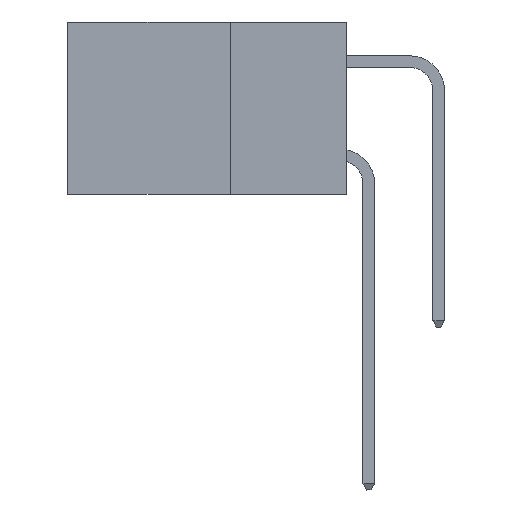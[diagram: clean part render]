
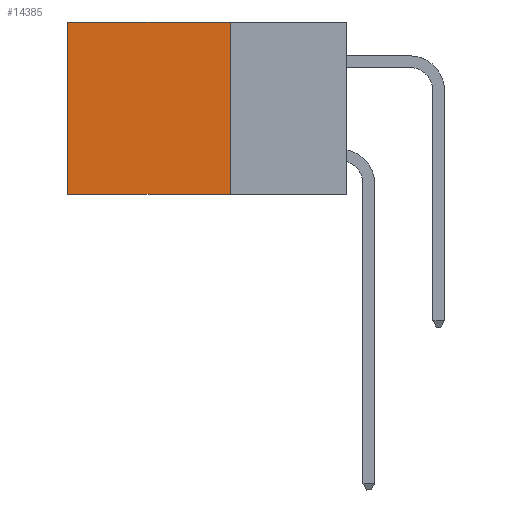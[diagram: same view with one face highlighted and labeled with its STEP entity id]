
A CAD part, left-side view. The second image highlights one B-rep face of the part: STEP entity #14385.
In plain terms, the highlighted planar face has unit normal (-1, 0, 0).
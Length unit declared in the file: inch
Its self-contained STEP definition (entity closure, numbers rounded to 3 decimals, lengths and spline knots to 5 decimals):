
#94 = CARTESIAN_POINT ( 'NONE',  ( 0.2875, 0.25, 0. ) ) ;
#2860 = DIRECTION ( 'NONE',  ( 0., 0., -1. ) ) ;
#2896 = ORIENTED_EDGE ( 'NONE', *, *, #21479, .T. ) ;
#3396 = EDGE_CURVE ( 'NONE', #15902, #11351, #21420, .T. ) ;
#3642 = DIRECTION ( 'NONE',  ( 0., 1., 0. ) ) ;
#4456 = CARTESIAN_POINT ( 'NONE',  ( 0.2875, 0.25, 0. ) ) ;
#4627 = CARTESIAN_POINT ( 'NONE',  ( 0.2875, 0.6, 0. ) ) ;
#4757 = VERTEX_POINT ( 'NONE', #4627 ) ;
#4791 = CARTESIAN_POINT ( 'NONE',  ( 0.2875, 0.25, -0.37 ) ) ;
#4839 = VERTEX_POINT ( 'NONE', #94 ) ;
#5002 = AXIS2_PLACEMENT_3D ( 'NONE', #4456, #22032, #11767 ) ;
#5581 = EDGE_LOOP ( 'NONE', ( #2896, #14275, #15285, #17978 ) ) ;
#5645 = LINE ( 'NONE', #17082, #9320 ) ;
#6939 = CARTESIAN_POINT ( 'NONE',  ( 0.2875, 0.25, 0. ) ) ;
#8459 = EDGE_CURVE ( 'NONE', #4839, #15902, #5645, .T. ) ;
#8718 = DIRECTION ( 'NONE',  ( 0., 1., 0. ) ) ;
#9116 = CARTESIAN_POINT ( 'NONE',  ( 0.2875, 0.25, -0.37 ) ) ;
#9320 = VECTOR ( 'NONE', #2860, 39.37008 ) ;
#9690 = CARTESIAN_POINT ( 'NONE',  ( 0.2875, 0.6, 0. ) ) ;
#9973 = PLANE ( 'NONE',  #5002 ) ;
#10730 = LINE ( 'NONE', #6939, #19358 ) ;
#11351 = VERTEX_POINT ( 'NONE', #12618 ) ;
#11506 = DIRECTION ( 'NONE',  ( 0., 0., -1. ) ) ;
#11767 = DIRECTION ( 'NONE',  ( 0., 0., -1. ) ) ;
#12109 = VECTOR ( 'NONE', #11506, 39.37008 ) ;
#12618 = CARTESIAN_POINT ( 'NONE',  ( 0.2875, 0.6, -0.37 ) ) ;
#14275 = ORIENTED_EDGE ( 'NONE', *, *, #3396, .F. ) ;
#14385 = ADVANCED_FACE ( 'NONE', ( #20444 ), #9973, .F. ) ;
#15285 = ORIENTED_EDGE ( 'NONE', *, *, #8459, .F. ) ;
#15750 = VECTOR ( 'NONE', #3642, 39.37008 ) ;
#15902 = VERTEX_POINT ( 'NONE', #9116 ) ;
#17082 = CARTESIAN_POINT ( 'NONE',  ( 0.2875, 0.25, 0. ) ) ;
#17978 = ORIENTED_EDGE ( 'NONE', *, *, #21776, .T. ) ;
#19358 = VECTOR ( 'NONE', #8718, 39.37008 ) ;
#20444 = FACE_OUTER_BOUND ( 'NONE', #5581, .T. ) ;
#21226 = LINE ( 'NONE', #9690, #12109 ) ;
#21420 = LINE ( 'NONE', #4791, #15750 ) ;
#21479 = EDGE_CURVE ( 'NONE', #4757, #11351, #21226, .T. ) ;
#21776 = EDGE_CURVE ( 'NONE', #4839, #4757, #10730, .T. ) ;
#22032 = DIRECTION ( 'NONE',  ( 1., 0., 0. ) ) ;
